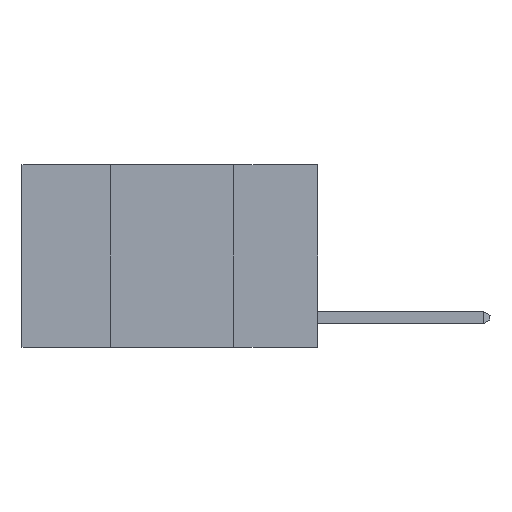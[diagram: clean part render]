
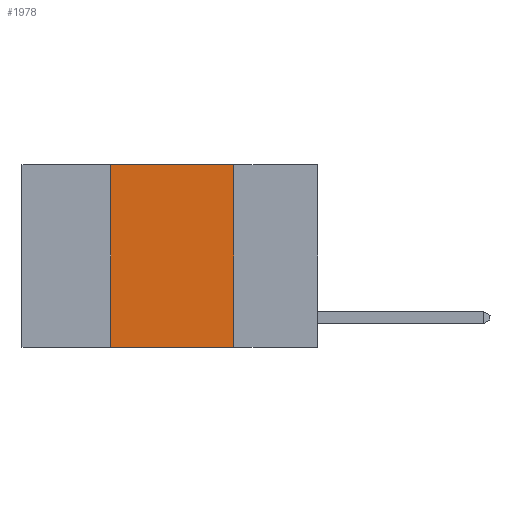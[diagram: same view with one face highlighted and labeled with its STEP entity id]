
A CAD part, left-side view. The second image highlights one B-rep face of the part: STEP entity #1978.
In plain terms, the highlighted planar face has unit normal (-1, 0, 0).
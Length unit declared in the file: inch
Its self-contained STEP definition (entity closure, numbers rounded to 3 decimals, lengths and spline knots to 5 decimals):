
#68 = VERTEX_POINT ( 'NONE', #6955 ) ;
#180 = VERTEX_POINT ( 'NONE', #5616 ) ;
#322 = DIRECTION ( 'NONE',  ( 1., 0., 0. ) ) ;
#636 = CARTESIAN_POINT ( 'NONE',  ( 0., 0.17, 0. ) ) ;
#930 = LINE ( 'NONE', #3141, #9041 ) ;
#1405 = DIRECTION ( 'NONE',  ( 0., 0., -1. ) ) ;
#1646 = EDGE_LOOP ( 'NONE', ( #6181, #2814, #7993, #4601 ) ) ;
#1903 = DIRECTION ( 'NONE',  ( 0., 0., -1. ) ) ;
#1978 = ADVANCED_FACE ( 'NONE', ( #5077 ), #8201, .F. ) ;
#2814 = ORIENTED_EDGE ( 'NONE', *, *, #5890, .F. ) ;
#3141 = CARTESIAN_POINT ( 'NONE',  ( 0., 0.6, 0. ) ) ;
#3457 = VERTEX_POINT ( 'NONE', #7829 ) ;
#3806 = LINE ( 'NONE', #636, #9927 ) ;
#4038 = CARTESIAN_POINT ( 'NONE',  ( 0., 0.42, -0.37 ) ) ;
#4212 = CARTESIAN_POINT ( 'NONE',  ( 0., 0.6, 0. ) ) ;
#4601 = ORIENTED_EDGE ( 'NONE', *, *, #8789, .T. ) ;
#4924 = VECTOR ( 'NONE', #10104, 39.37008 ) ;
#4968 = DIRECTION ( 'NONE',  ( 0., -1., 0. ) ) ;
#5077 = FACE_OUTER_BOUND ( 'NONE', #1646, .T. ) ;
#5616 = CARTESIAN_POINT ( 'NONE',  ( 0., 0.42, 0. ) ) ;
#5890 = EDGE_CURVE ( 'NONE', #180, #68, #930, .T. ) ;
#6181 = ORIENTED_EDGE ( 'NONE', *, *, #8577, .F. ) ;
#6227 = LINE ( 'NONE', #7687, #4924 ) ;
#6229 = EDGE_CURVE ( 'NONE', #9590, #180, #6227, .T. ) ;
#6290 = DIRECTION ( 'NONE',  ( 0., -1., 0. ) ) ;
#6955 = CARTESIAN_POINT ( 'NONE',  ( 0., 0.17, 0. ) ) ;
#7274 = VECTOR ( 'NONE', #4968, 39.37008 ) ;
#7687 = CARTESIAN_POINT ( 'NONE',  ( 0., 0.42, 0. ) ) ;
#7829 = CARTESIAN_POINT ( 'NONE',  ( 0., 0.17, -0.37 ) ) ;
#7977 = AXIS2_PLACEMENT_3D ( 'NONE', #4212, #322, #1903 ) ;
#7993 = ORIENTED_EDGE ( 'NONE', *, *, #6229, .F. ) ;
#8201 = PLANE ( 'NONE',  #7977 ) ;
#8577 = EDGE_CURVE ( 'NONE', #68, #3457, #3806, .T. ) ;
#8789 = EDGE_CURVE ( 'NONE', #9590, #3457, #9635, .T. ) ;
#8867 = CARTESIAN_POINT ( 'NONE',  ( 0., 0.6, -0.37 ) ) ;
#9041 = VECTOR ( 'NONE', #6290, 39.37008 ) ;
#9590 = VERTEX_POINT ( 'NONE', #4038 ) ;
#9635 = LINE ( 'NONE', #8867, #7274 ) ;
#9927 = VECTOR ( 'NONE', #1405, 39.37008 ) ;
#10104 = DIRECTION ( 'NONE',  ( 0., 0., 1. ) ) ;
